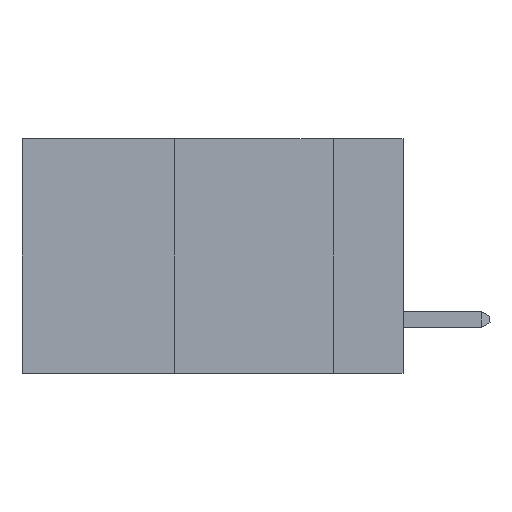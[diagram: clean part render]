
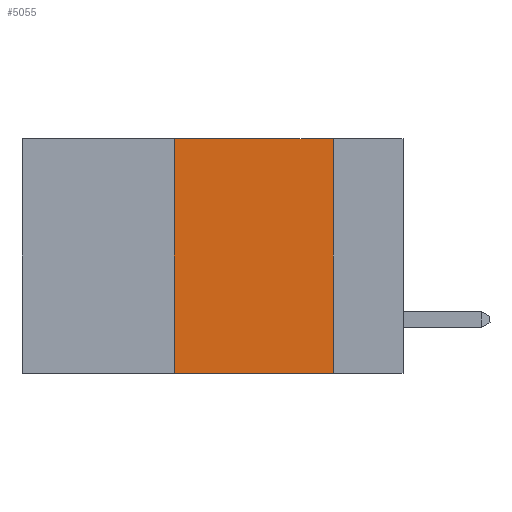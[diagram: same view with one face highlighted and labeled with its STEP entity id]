
A CAD part, left-side view. The second image highlights one B-rep face of the part: STEP entity #5055.
In plain terms, the highlighted planar face has unit normal (-1, 0, 0).
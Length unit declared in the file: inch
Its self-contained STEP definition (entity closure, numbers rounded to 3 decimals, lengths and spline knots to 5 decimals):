
#150 = ORIENTED_EDGE ( 'NONE', *, *, #3037, .F. ) ;
#669 = CARTESIAN_POINT ( 'NONE',  ( 0., 0.6, 0. ) ) ;
#1101 = VECTOR ( 'NONE', #15347, 39.37008 ) ;
#1334 = EDGE_LOOP ( 'NONE', ( #2029, #150, #11106, #6922 ) ) ;
#2029 = ORIENTED_EDGE ( 'NONE', *, *, #13129, .F. ) ;
#3037 = EDGE_CURVE ( 'NONE', #12558, #9178, #18174, .T. ) ;
#4850 = CARTESIAN_POINT ( 'NONE',  ( 0., 0.6, 0. ) ) ;
#5055 = ADVANCED_FACE ( 'NONE', ( #20915 ), #17530, .F. ) ;
#5321 = VECTOR ( 'NONE', #20610, 39.37008 ) ;
#6255 = CARTESIAN_POINT ( 'NONE',  ( 0., 0.36, 0. ) ) ;
#6302 = CARTESIAN_POINT ( 'NONE',  ( 0., 0.36, -0.37 ) ) ;
#6922 = ORIENTED_EDGE ( 'NONE', *, *, #20277, .T. ) ;
#7580 = VERTEX_POINT ( 'NONE', #12111 ) ;
#8654 = DIRECTION ( 'NONE',  ( 0., 0., -1. ) ) ;
#9178 = VERTEX_POINT ( 'NONE', #13606 ) ;
#9244 = LINE ( 'NONE', #13872, #18147 ) ;
#9998 = DIRECTION ( 'NONE',  ( 0., -1., 0. ) ) ;
#11106 = ORIENTED_EDGE ( 'NONE', *, *, #21487, .F. ) ;
#12089 = AXIS2_PLACEMENT_3D ( 'NONE', #4850, #19340, #8654 ) ;
#12111 = CARTESIAN_POINT ( 'NONE',  ( 0., 0.11, -0.37 ) ) ;
#12558 = VERTEX_POINT ( 'NONE', #18875 ) ;
#13129 = EDGE_CURVE ( 'NONE', #9178, #7580, #15539, .T. ) ;
#13606 = CARTESIAN_POINT ( 'NONE',  ( 0., 0.11, 0. ) ) ;
#13872 = CARTESIAN_POINT ( 'NONE',  ( 0., 0.6, -0.37 ) ) ;
#14672 = LINE ( 'NONE', #6255, #1101 ) ;
#15347 = DIRECTION ( 'NONE',  ( 0., 0., 1. ) ) ;
#15539 = LINE ( 'NONE', #18766, #5321 ) ;
#15628 = DIRECTION ( 'NONE',  ( 0., -1., 0. ) ) ;
#16010 = VERTEX_POINT ( 'NONE', #6302 ) ;
#17530 = PLANE ( 'NONE',  #12089 ) ;
#17623 = VECTOR ( 'NONE', #9998, 39.37008 ) ;
#18147 = VECTOR ( 'NONE', #15628, 39.37008 ) ;
#18174 = LINE ( 'NONE', #669, #17623 ) ;
#18766 = CARTESIAN_POINT ( 'NONE',  ( 0., 0.11, 0. ) ) ;
#18875 = CARTESIAN_POINT ( 'NONE',  ( 0., 0.36, 0. ) ) ;
#19340 = DIRECTION ( 'NONE',  ( 1., 0., 0. ) ) ;
#20277 = EDGE_CURVE ( 'NONE', #16010, #7580, #9244, .T. ) ;
#20610 = DIRECTION ( 'NONE',  ( 0., 0., -1. ) ) ;
#20915 = FACE_OUTER_BOUND ( 'NONE', #1334, .T. ) ;
#21487 = EDGE_CURVE ( 'NONE', #16010, #12558, #14672, .T. ) ;
